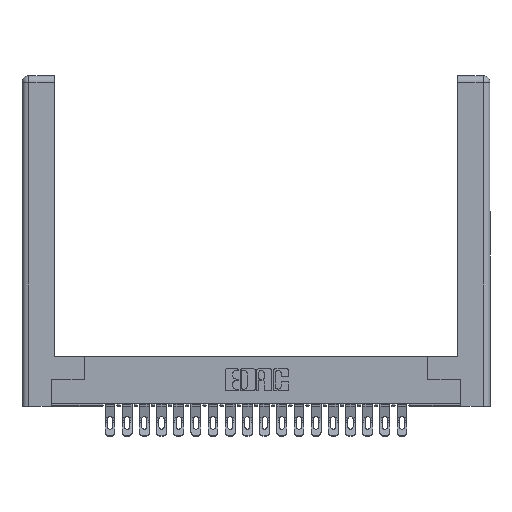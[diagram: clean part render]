
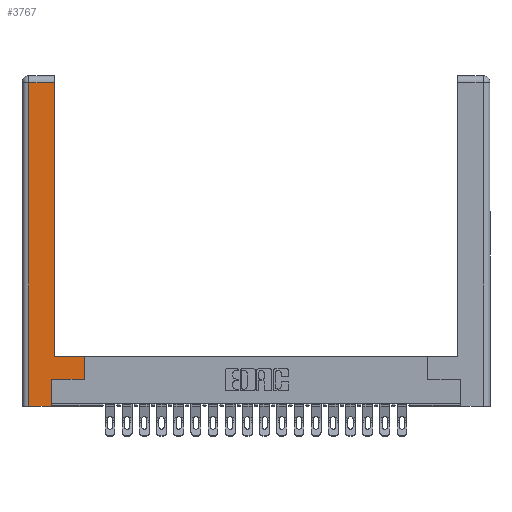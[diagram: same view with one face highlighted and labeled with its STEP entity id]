
A CAD part, top view. The second image highlights one B-rep face of the part: STEP entity #3767.
In plain terms, the highlighted planar face has unit normal (0, 0, 1).
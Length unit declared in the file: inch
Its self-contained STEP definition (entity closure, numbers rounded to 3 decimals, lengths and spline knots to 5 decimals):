
#123 = DIRECTION ( 'NONE',  ( -1., 0., 0. ) ) ;
#389 = AXIS2_PLACEMENT_3D ( 'NONE', #1521, #9413, #9320 ) ;
#407 = CARTESIAN_POINT ( 'NONE',  ( 0.0615, 2.94, 0. ) ) ;
#442 = ORIENTED_EDGE ( 'NONE', *, *, #9903, .T. ) ;
#1195 = VERTEX_POINT ( 'NONE', #407 ) ;
#1521 = CARTESIAN_POINT ( 'NONE',  ( 0., 0., 0. ) ) ;
#1878 = EDGE_LOOP ( 'NONE', ( #5670, #18240, #8984, #442, #7301, #10769, #16948, #7096 ) ) ;
#2132 = LINE ( 'NONE', #4393, #16034 ) ;
#2173 = DIRECTION ( 'NONE',  ( 1., 0., 0. ) ) ;
#2488 = LINE ( 'NONE', #3840, #18547 ) ;
#2586 = LINE ( 'NONE', #19881, #10017 ) ;
#2613 = VECTOR ( 'NONE', #15594, 39.37008 ) ;
#3016 = VERTEX_POINT ( 'NONE', #13509 ) ;
#3594 = DIRECTION ( 'NONE',  ( 0., 1., 0. ) ) ;
#3767 = ADVANCED_FACE ( 'NONE', ( #13147 ), #13561, .F. ) ;
#3797 = VERTEX_POINT ( 'NONE', #21160 ) ;
#3831 = EDGE_CURVE ( 'NONE', #3016, #3797, #14670, .T. ) ;
#3840 = CARTESIAN_POINT ( 'NONE',  ( 0.565, 0.245, 0. ) ) ;
#4023 = VERTEX_POINT ( 'NONE', #6207 ) ;
#4393 = CARTESIAN_POINT ( 'NONE',  ( 0.0615, 2.94, 0. ) ) ;
#5670 = ORIENTED_EDGE ( 'NONE', *, *, #11558, .T. ) ;
#6207 = CARTESIAN_POINT ( 'NONE',  ( 0.265, 0., 0. ) ) ;
#6954 = EDGE_CURVE ( 'NONE', #21593, #1195, #2132, .T. ) ;
#7096 = ORIENTED_EDGE ( 'NONE', *, *, #22683, .T. ) ;
#7301 = ORIENTED_EDGE ( 'NONE', *, *, #8172, .T. ) ;
#8172 = EDGE_CURVE ( 'NONE', #4023, #14056, #16282, .T. ) ;
#8765 = CARTESIAN_POINT ( 'NONE',  ( 0.295, 3., 0. ) ) ;
#8984 = ORIENTED_EDGE ( 'NONE', *, *, #9900, .T. ) ;
#9320 = DIRECTION ( 'NONE',  ( -1., 0., 0. ) ) ;
#9413 = DIRECTION ( 'NONE',  ( 0., 0., -1. ) ) ;
#9834 = DIRECTION ( 'NONE',  ( 1., 0., 0. ) ) ;
#9900 = EDGE_CURVE ( 'NONE', #1195, #18950, #22401, .T. ) ;
#9903 = EDGE_CURVE ( 'NONE', #18950, #4023, #2586, .T. ) ;
#10017 = VECTOR ( 'NONE', #2173, 39.37008 ) ;
#10497 = CARTESIAN_POINT ( 'NONE',  ( 0.265, 0.245, 0. ) ) ;
#10769 = ORIENTED_EDGE ( 'NONE', *, *, #19225, .T. ) ;
#11558 = EDGE_CURVE ( 'NONE', #24386, #21593, #21668, .T. ) ;
#11787 = CARTESIAN_POINT ( 'NONE',  ( 0.0615, 0., 0. ) ) ;
#13147 = FACE_OUTER_BOUND ( 'NONE', #1878, .T. ) ;
#13309 = CARTESIAN_POINT ( 'NONE',  ( 0.565, 0.45, 0. ) ) ;
#13509 = CARTESIAN_POINT ( 'NONE',  ( 0.565, 0.245, 0. ) ) ;
#13561 = PLANE ( 'NONE',  #389 ) ;
#13699 = CARTESIAN_POINT ( 'NONE',  ( 0.295, 0.45, 0. ) ) ;
#13916 = VECTOR ( 'NONE', #16723, 39.37008 ) ;
#14056 = VERTEX_POINT ( 'NONE', #15435 ) ;
#14670 = LINE ( 'NONE', #13309, #18669 ) ;
#15435 = CARTESIAN_POINT ( 'NONE',  ( 0.265, 0.245, 0. ) ) ;
#15594 = DIRECTION ( 'NONE',  ( -1., 0., 0. ) ) ;
#16034 = VECTOR ( 'NONE', #123, 39.37008 ) ;
#16271 = DIRECTION ( 'NONE',  ( 0., 1., 0. ) ) ;
#16282 = LINE ( 'NONE', #10497, #23125 ) ;
#16723 = DIRECTION ( 'NONE',  ( 0., 1., 0. ) ) ;
#16797 = VECTOR ( 'NONE', #21805, 39.37008 ) ;
#16948 = ORIENTED_EDGE ( 'NONE', *, *, #3831, .T. ) ;
#17654 = CARTESIAN_POINT ( 'NONE',  ( 0.295, 2.94, 0. ) ) ;
#18240 = ORIENTED_EDGE ( 'NONE', *, *, #6954, .T. ) ;
#18398 = LINE ( 'NONE', #25493, #2613 ) ;
#18547 = VECTOR ( 'NONE', #9834, 39.37008 ) ;
#18669 = VECTOR ( 'NONE', #3594, 39.37008 ) ;
#18950 = VERTEX_POINT ( 'NONE', #22894 ) ;
#19225 = EDGE_CURVE ( 'NONE', #14056, #3016, #2488, .T. ) ;
#19881 = CARTESIAN_POINT ( 'NONE',  ( 0.265, 0., 0. ) ) ;
#21160 = CARTESIAN_POINT ( 'NONE',  ( 0.565, 0.45, 0. ) ) ;
#21593 = VERTEX_POINT ( 'NONE', #17654 ) ;
#21668 = LINE ( 'NONE', #8765, #13916 ) ;
#21805 = DIRECTION ( 'NONE',  ( 0., -1., 0. ) ) ;
#22401 = LINE ( 'NONE', #11787, #16797 ) ;
#22683 = EDGE_CURVE ( 'NONE', #3797, #24386, #18398, .T. ) ;
#22894 = CARTESIAN_POINT ( 'NONE',  ( 0.0615, 0., 0. ) ) ;
#23125 = VECTOR ( 'NONE', #16271, 39.37008 ) ;
#24386 = VERTEX_POINT ( 'NONE', #13699 ) ;
#25493 = CARTESIAN_POINT ( 'NONE',  ( 0.295, 0.45, 0. ) ) ;
